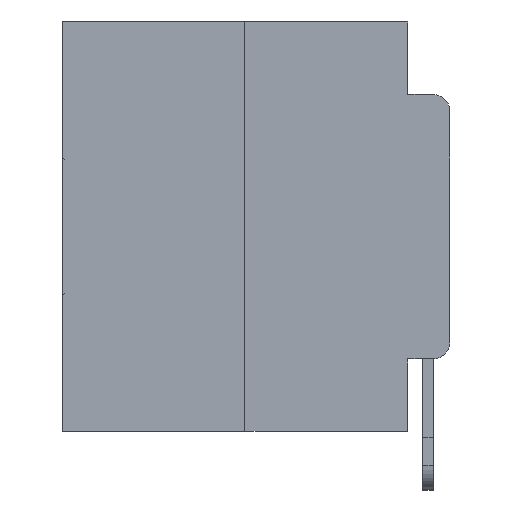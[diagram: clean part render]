
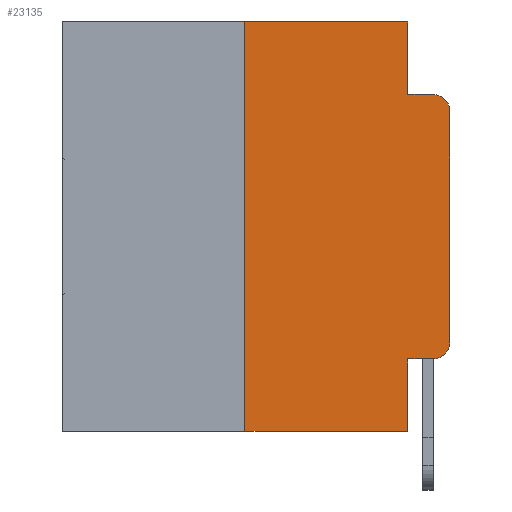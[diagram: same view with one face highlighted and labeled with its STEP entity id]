
A CAD part, left-side view. The second image highlights one B-rep face of the part: STEP entity #23135.
In plain terms, the highlighted planar face has unit normal (-1, 0, 0).
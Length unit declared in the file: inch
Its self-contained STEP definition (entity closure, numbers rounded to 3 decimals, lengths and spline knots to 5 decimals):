
#438 = EDGE_CURVE ( 'NONE', #7836, #19099, #20611, .T. ) ;
#492 = LINE ( 'NONE', #12458, #5276 ) ;
#577 = EDGE_CURVE ( 'NONE', #4691, #28465, #17139, .T. ) ;
#656 = EDGE_LOOP ( 'NONE', ( #8446, #1618, #10554, #24156, #10931, #9535, #9172, #19700, #9927, #4275 ) ) ;
#1063 = PLANE ( 'NONE',  #24913 ) ;
#1441 = CARTESIAN_POINT ( 'NONE',  ( 0., 0.051, -0.4115 ) ) ;
#1618 = ORIENTED_EDGE ( 'NONE', *, *, #7898, .T. ) ;
#2138 = DIRECTION ( 'NONE',  ( 0., 0., -1. ) ) ;
#2216 = LINE ( 'NONE', #16615, #6900 ) ;
#3021 = DIRECTION ( 'NONE',  ( -1., 0., 0. ) ) ;
#3455 = DIRECTION ( 'NONE',  ( 0., 0., 1. ) ) ;
#3627 = CARTESIAN_POINT ( 'NONE',  ( 0., 0., -0.1085 ) ) ;
#3642 = EDGE_CURVE ( 'NONE', #19099, #21786, #5247, .T. ) ;
#3809 = VECTOR ( 'NONE', #2138, 39.37008 ) ;
#4261 = CARTESIAN_POINT ( 'NONE',  ( 0., 0.051, -0.5 ) ) ;
#4275 = ORIENTED_EDGE ( 'NONE', *, *, #23484, .T. ) ;
#4619 = CARTESIAN_POINT ( 'NONE',  ( 0., 0.051, 0. ) ) ;
#4691 = VERTEX_POINT ( 'NONE', #1441 ) ;
#5247 = LINE ( 'NONE', #26765, #3809 ) ;
#5276 = VECTOR ( 'NONE', #3455, 39.37008 ) ;
#5350 = CARTESIAN_POINT ( 'NONE',  ( 0., 0.02, -0.4115 ) ) ;
#5455 = DIRECTION ( 'NONE',  ( 0., 0., 1. ) ) ;
#5476 = VECTOR ( 'NONE', #19569, 39.37008 ) ;
#5494 = EDGE_CURVE ( 'NONE', #25934, #23353, #20199, .T. ) ;
#5543 = EDGE_CURVE ( 'NONE', #21786, #25450, #23983, .T. ) ;
#6536 = VERTEX_POINT ( 'NONE', #16119 ) ;
#6900 = VECTOR ( 'NONE', #5455, 39.37008 ) ;
#7092 = CIRCLE ( 'NONE', #22975, 0.02 ) ;
#7836 = VERTEX_POINT ( 'NONE', #9462 ) ;
#7898 = EDGE_CURVE ( 'NONE', #16074, #25450, #7092, .T. ) ;
#8036 = CARTESIAN_POINT ( 'NONE',  ( 0., 0.473, 0. ) ) ;
#8446 = ORIENTED_EDGE ( 'NONE', *, *, #15943, .T. ) ;
#9172 = ORIENTED_EDGE ( 'NONE', *, *, #5494, .T. ) ;
#9191 = DIRECTION ( 'NONE',  ( -1., 0., 0. ) ) ;
#9206 = CARTESIAN_POINT ( 'NONE',  ( 0., 0.473, 0. ) ) ;
#9435 = VECTOR ( 'NONE', #12958, 39.37008 ) ;
#9462 = CARTESIAN_POINT ( 'NONE',  ( 0., 0.25, 0. ) ) ;
#9535 = ORIENTED_EDGE ( 'NONE', *, *, #25052, .F. ) ;
#9927 = ORIENTED_EDGE ( 'NONE', *, *, #577, .T. ) ;
#10285 = DIRECTION ( 'NONE',  ( 0., 0., -1. ) ) ;
#10554 = ORIENTED_EDGE ( 'NONE', *, *, #5543, .F. ) ;
#10876 = CARTESIAN_POINT ( 'NONE',  ( 0., 0.25, -0.5 ) ) ;
#10931 = ORIENTED_EDGE ( 'NONE', *, *, #438, .F. ) ;
#12158 = LINE ( 'NONE', #25752, #5476 ) ;
#12177 = VECTOR ( 'NONE', #26751, 39.37008 ) ;
#12458 = CARTESIAN_POINT ( 'NONE',  ( 0., 0.25, 0. ) ) ;
#12958 = DIRECTION ( 'NONE',  ( 0., -1., 0. ) ) ;
#13466 = CARTESIAN_POINT ( 'NONE',  ( 0., 0.051, -0.0885 ) ) ;
#13555 = DIRECTION ( 'NONE',  ( 0., -1., 0. ) ) ;
#13606 = VECTOR ( 'NONE', #24408, 39.37008 ) ;
#15901 = FACE_OUTER_BOUND ( 'NONE', #656, .T. ) ;
#15943 = EDGE_CURVE ( 'NONE', #6536, #16074, #2216, .T. ) ;
#16074 = VERTEX_POINT ( 'NONE', #3627 ) ;
#16119 = CARTESIAN_POINT ( 'NONE',  ( 0., 0., -0.3915 ) ) ;
#16446 = VECTOR ( 'NONE', #13555, 39.37008 ) ;
#16523 = CARTESIAN_POINT ( 'NONE',  ( 0., 0.02, -0.1085 ) ) ;
#16615 = CARTESIAN_POINT ( 'NONE',  ( 0., 0., 0. ) ) ;
#17139 = LINE ( 'NONE', #28040, #16446 ) ;
#18429 = AXIS2_PLACEMENT_3D ( 'NONE', #22549, #9191, #24779 ) ;
#18765 = DIRECTION ( 'NONE',  ( 0., 0., -1. ) ) ;
#19099 = VERTEX_POINT ( 'NONE', #4619 ) ;
#19569 = DIRECTION ( 'NONE',  ( 0., 0., -1. ) ) ;
#19700 = ORIENTED_EDGE ( 'NONE', *, *, #29159, .F. ) ;
#20199 = LINE ( 'NONE', #22187, #13606 ) ;
#20611 = LINE ( 'NONE', #9206, #9435 ) ;
#21786 = VERTEX_POINT ( 'NONE', #26421 ) ;
#22187 = CARTESIAN_POINT ( 'NONE',  ( 0., 0.473, -0.5 ) ) ;
#22549 = CARTESIAN_POINT ( 'NONE',  ( 0., 0.02, -0.3915 ) ) ;
#22975 = AXIS2_PLACEMENT_3D ( 'NONE', #16523, #3021, #18765 ) ;
#23135 = ADVANCED_FACE ( 'NONE', ( #15901 ), #1063, .F. ) ;
#23353 = VERTEX_POINT ( 'NONE', #4261 ) ;
#23484 = EDGE_CURVE ( 'NONE', #28465, #6536, #25229, .T. ) ;
#23629 = DIRECTION ( 'NONE',  ( 1., 0., 0. ) ) ;
#23983 = LINE ( 'NONE', #13466, #12177 ) ;
#24156 = ORIENTED_EDGE ( 'NONE', *, *, #3642, .F. ) ;
#24408 = DIRECTION ( 'NONE',  ( 0., -1., 0. ) ) ;
#24779 = DIRECTION ( 'NONE',  ( 0., 0., -1. ) ) ;
#24913 = AXIS2_PLACEMENT_3D ( 'NONE', #8036, #23629, #10285 ) ;
#25052 = EDGE_CURVE ( 'NONE', #25934, #7836, #492, .T. ) ;
#25229 = CIRCLE ( 'NONE', #18429, 0.02 ) ;
#25450 = VERTEX_POINT ( 'NONE', #27187 ) ;
#25752 = CARTESIAN_POINT ( 'NONE',  ( 0., 0.051, 0. ) ) ;
#25934 = VERTEX_POINT ( 'NONE', #10876 ) ;
#26421 = CARTESIAN_POINT ( 'NONE',  ( 0., 0.051, -0.0885 ) ) ;
#26751 = DIRECTION ( 'NONE',  ( 0., -1., 0. ) ) ;
#26765 = CARTESIAN_POINT ( 'NONE',  ( 0., 0.051, 0. ) ) ;
#27187 = CARTESIAN_POINT ( 'NONE',  ( 0., 0.02, -0.0885 ) ) ;
#28040 = CARTESIAN_POINT ( 'NONE',  ( 0., 0.051, -0.4115 ) ) ;
#28465 = VERTEX_POINT ( 'NONE', #5350 ) ;
#29159 = EDGE_CURVE ( 'NONE', #4691, #23353, #12158, .T. ) ;
